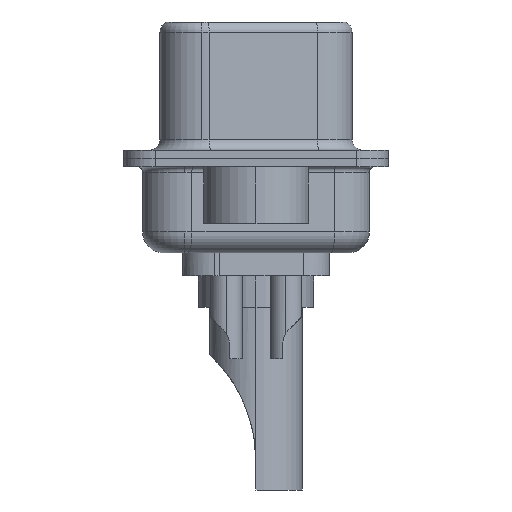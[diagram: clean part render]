
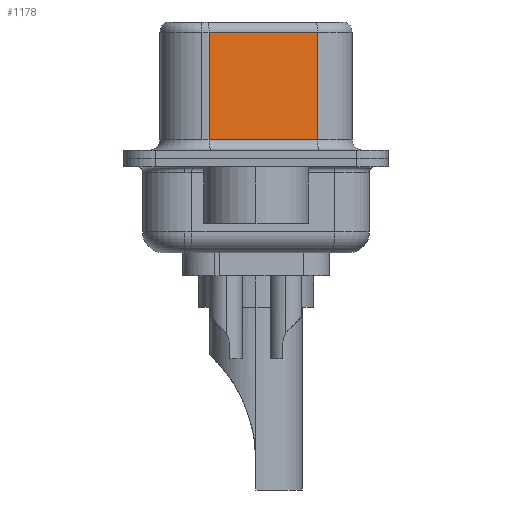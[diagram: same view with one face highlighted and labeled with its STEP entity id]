
A CAD part, left-side view. The second image highlights one B-rep face of the part: STEP entity #1178.
In plain terms, the highlighted planar face has unit normal (-0.985, -0.174, 0).
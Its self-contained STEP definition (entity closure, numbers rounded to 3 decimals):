
#259 = CARTESIAN_POINT ( 'NONE',  ( 4.565, -2.927, 6.02 ) ) ;
#932 = ORIENTED_EDGE ( 'NONE', *, *, #3339, .T. ) ;
#1152 = CARTESIAN_POINT ( 'NONE',  ( 4.565, -2.927, 6.02 ) ) ;
#1178 = ADVANCED_FACE ( 'NONE', ( #16121 ), #2274, .F. ) ;
#1417 = CARTESIAN_POINT ( 'NONE',  ( 3.655, 2.233, 6.02 ) ) ;
#1852 = DIRECTION ( 'NONE',  ( 0., 0., -1. ) ) ;
#2264 = CARTESIAN_POINT ( 'NONE',  ( 3.655, 2.233, 0.9 ) ) ;
#2274 = PLANE ( 'NONE',  #14669 ) ;
#3159 = EDGE_CURVE ( 'NONE', #10177, #8049, #12760, .T. ) ;
#3339 = EDGE_CURVE ( 'NONE', #11965, #10177, #6281, .T. ) ;
#4088 = EDGE_CURVE ( 'NONE', #15637, #8049, #16233, .T. ) ;
#5208 = VECTOR ( 'NONE', #9099, 1000. ) ;
#5623 = VECTOR ( 'NONE', #1852, 1000. ) ;
#6164 = CARTESIAN_POINT ( 'NONE',  ( 4.565, -2.927, 0.9 ) ) ;
#6281 = LINE ( 'NONE', #15004, #12946 ) ;
#7747 = CARTESIAN_POINT ( 'NONE',  ( 4.565, -2.927, 0.9 ) ) ;
#8049 = VERTEX_POINT ( 'NONE', #7747 ) ;
#8162 = EDGE_CURVE ( 'NONE', #15637, #11965, #12809, .T. ) ;
#9099 = DIRECTION ( 'NONE',  ( 0.174, -0.985, 0. ) ) ;
#9383 = CARTESIAN_POINT ( 'NONE',  ( 4.565, -2.927, 6.52 ) ) ;
#10177 = VERTEX_POINT ( 'NONE', #2264 ) ;
#11024 = CARTESIAN_POINT ( 'NONE',  ( 4.565, -2.927, 6.52 ) ) ;
#11048 = EDGE_LOOP ( 'NONE', ( #14838, #14819, #932, #16120 ) ) ;
#11965 = VERTEX_POINT ( 'NONE', #1417 ) ;
#12008 = DIRECTION ( 'NONE',  ( -0.174, 0.985, 0. ) ) ;
#12760 = LINE ( 'NONE', #6164, #5208 ) ;
#12809 = LINE ( 'NONE', #1152, #15911 ) ;
#12946 = VECTOR ( 'NONE', #17302, 1000. ) ;
#14669 = AXIS2_PLACEMENT_3D ( 'NONE', #9383, #17361, #14958 ) ;
#14819 = ORIENTED_EDGE ( 'NONE', *, *, #8162, .T. ) ;
#14838 = ORIENTED_EDGE ( 'NONE', *, *, #4088, .F. ) ;
#14958 = DIRECTION ( 'NONE',  ( -0.174, 0.985, 0. ) ) ;
#15004 = CARTESIAN_POINT ( 'NONE',  ( 3.655, 2.233, 6.52 ) ) ;
#15637 = VERTEX_POINT ( 'NONE', #259 ) ;
#15911 = VECTOR ( 'NONE', #12008, 1000. ) ;
#16120 = ORIENTED_EDGE ( 'NONE', *, *, #3159, .T. ) ;
#16121 = FACE_OUTER_BOUND ( 'NONE', #11048, .T. ) ;
#16233 = LINE ( 'NONE', #11024, #5623 ) ;
#17302 = DIRECTION ( 'NONE',  ( 0., 0., -1. ) ) ;
#17361 = DIRECTION ( 'NONE',  ( 0.985, 0.174, 0. ) ) ;
